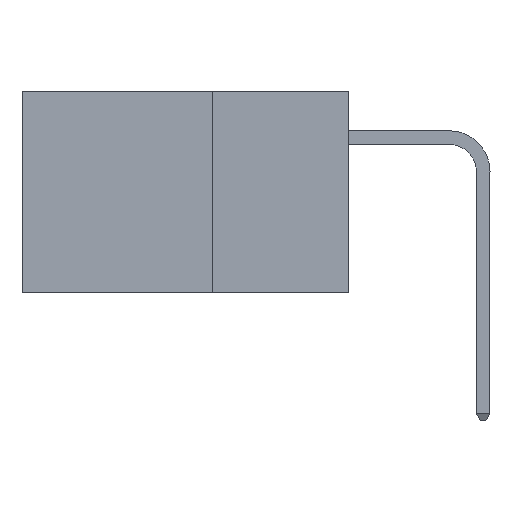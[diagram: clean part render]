
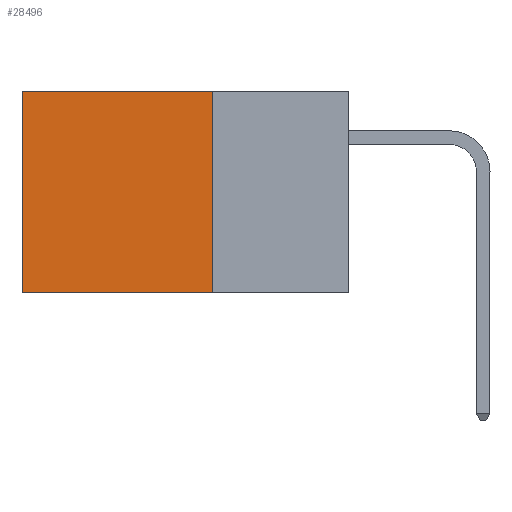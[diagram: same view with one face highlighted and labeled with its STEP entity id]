
A CAD part, left-side view. The second image highlights one B-rep face of the part: STEP entity #28496.
In plain terms, the highlighted planar face has unit normal (-1, 0, 0).
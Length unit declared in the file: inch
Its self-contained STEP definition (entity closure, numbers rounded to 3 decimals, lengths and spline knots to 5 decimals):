
#668 = ORIENTED_EDGE ( 'NONE', *, *, #30635, .F. ) ;
#2224 = DIRECTION ( 'NONE',  ( 0., 1., 0. ) ) ;
#2282 = AXIS2_PLACEMENT_3D ( 'NONE', #20371, #11703, #31850 ) ;
#5900 = CARTESIAN_POINT ( 'NONE',  ( 0.2875, 0.6, -0.37 ) ) ;
#6262 = VECTOR ( 'NONE', #36442, 39.37008 ) ;
#7189 = LINE ( 'NONE', #7603, #6262 ) ;
#7523 = VECTOR ( 'NONE', #8236, 39.37008 ) ;
#7603 = CARTESIAN_POINT ( 'NONE',  ( 0.2875, 0.6, 0. ) ) ;
#8044 = VERTEX_POINT ( 'NONE', #23404 ) ;
#8236 = DIRECTION ( 'NONE',  ( 0., 0., -1. ) ) ;
#8985 = VECTOR ( 'NONE', #2224, 39.37008 ) ;
#9128 = CARTESIAN_POINT ( 'NONE',  ( 0.2875, 0.6, 0. ) ) ;
#9994 = EDGE_CURVE ( 'NONE', #17421, #17338, #7189, .T. ) ;
#10120 = ORIENTED_EDGE ( 'NONE', *, *, #30683, .T. ) ;
#11703 = DIRECTION ( 'NONE',  ( 1., 0., 0. ) ) ;
#16812 = VECTOR ( 'NONE', #19734, 39.37008 ) ;
#17006 = FACE_OUTER_BOUND ( 'NONE', #35539, .T. ) ;
#17338 = VERTEX_POINT ( 'NONE', #5900 ) ;
#17421 = VERTEX_POINT ( 'NONE', #9128 ) ;
#19734 = DIRECTION ( 'NONE',  ( 0., 1., 0. ) ) ;
#20371 = CARTESIAN_POINT ( 'NONE',  ( 0.2875, 0.25, 0. ) ) ;
#20705 = ORIENTED_EDGE ( 'NONE', *, *, #36748, .F. ) ;
#23404 = CARTESIAN_POINT ( 'NONE',  ( 0.2875, 0.25, 0. ) ) ;
#24461 = LINE ( 'NONE', #28349, #8985 ) ;
#26134 = PLANE ( 'NONE',  #2282 ) ;
#27145 = LINE ( 'NONE', #33922, #16812 ) ;
#28349 = CARTESIAN_POINT ( 'NONE',  ( 0.2875, 0.25, 0. ) ) ;
#28404 = CARTESIAN_POINT ( 'NONE',  ( 0.2875, 0.25, 0. ) ) ;
#28496 = ADVANCED_FACE ( 'NONE', ( #17006 ), #26134, .F. ) ;
#30616 = LINE ( 'NONE', #28404, #7523 ) ;
#30635 = EDGE_CURVE ( 'NONE', #36563, #17338, #27145, .T. ) ;
#30683 = EDGE_CURVE ( 'NONE', #8044, #17421, #24461, .T. ) ;
#31850 = DIRECTION ( 'NONE',  ( 0., 0., -1. ) ) ;
#33878 = ORIENTED_EDGE ( 'NONE', *, *, #9994, .T. ) ;
#33922 = CARTESIAN_POINT ( 'NONE',  ( 0.2875, 0.25, -0.37 ) ) ;
#35539 = EDGE_LOOP ( 'NONE', ( #33878, #668, #20705, #10120 ) ) ;
#36213 = CARTESIAN_POINT ( 'NONE',  ( 0.2875, 0.25, -0.37 ) ) ;
#36442 = DIRECTION ( 'NONE',  ( 0., 0., -1. ) ) ;
#36563 = VERTEX_POINT ( 'NONE', #36213 ) ;
#36748 = EDGE_CURVE ( 'NONE', #8044, #36563, #30616, .T. ) ;
